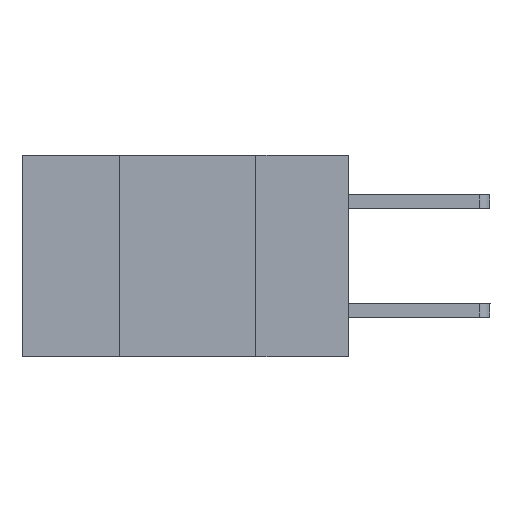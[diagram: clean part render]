
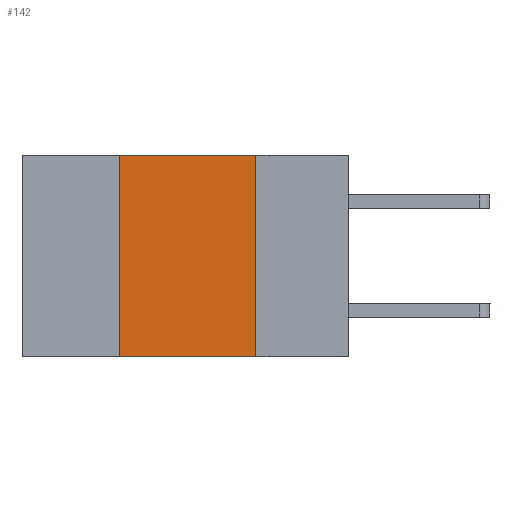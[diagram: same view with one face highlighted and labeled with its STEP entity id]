
A CAD part, left-side view. The second image highlights one B-rep face of the part: STEP entity #142.
In plain terms, the highlighted planar face has unit normal (-1, 0, 0).
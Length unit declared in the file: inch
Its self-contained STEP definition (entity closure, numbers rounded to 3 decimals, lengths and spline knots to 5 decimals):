
#65 = EDGE_CURVE ( 'NONE', #6121, #2360, #4379, .T. ) ;
#142 = ADVANCED_FACE ( 'NONE', ( #5683 ), #5788, .F. ) ;
#207 = LINE ( 'NONE', #7475, #9619 ) ;
#373 = EDGE_CURVE ( 'NONE', #6121, #1591, #207, .T. ) ;
#1591 = VERTEX_POINT ( 'NONE', #2227 ) ;
#1872 = CARTESIAN_POINT ( 'NONE',  ( 0., 0.17, -0.37 ) ) ;
#1943 = VECTOR ( 'NONE', #3594, 39.37008 ) ;
#2227 = CARTESIAN_POINT ( 'NONE',  ( 0., 0.42, 0. ) ) ;
#2360 = VERTEX_POINT ( 'NONE', #1872 ) ;
#2389 = VECTOR ( 'NONE', #4995, 39.37008 ) ;
#3249 = ORIENTED_EDGE ( 'NONE', *, *, #4396, .F. ) ;
#3594 = DIRECTION ( 'NONE',  ( 0., -1., 0. ) ) ;
#3815 = CARTESIAN_POINT ( 'NONE',  ( 0., 0.6, 0. ) ) ;
#3959 = CARTESIAN_POINT ( 'NONE',  ( 0., 0.17, -0.37 ) ) ;
#4371 = VECTOR ( 'NONE', #8391, 39.37008 ) ;
#4379 = LINE ( 'NONE', #9118, #2389 ) ;
#4396 = EDGE_CURVE ( 'NONE', #1591, #7978, #6060, .T. ) ;
#4505 = CARTESIAN_POINT ( 'NONE',  ( 0., 0.17, 0. ) ) ;
#4606 = DIRECTION ( 'NONE',  ( 0., 0., -1. ) ) ;
#4995 = DIRECTION ( 'NONE',  ( 0., -1., 0. ) ) ;
#5183 = DIRECTION ( 'NONE',  ( 0., 0., 1. ) ) ;
#5683 = FACE_OUTER_BOUND ( 'NONE', #9053, .T. ) ;
#5733 = AXIS2_PLACEMENT_3D ( 'NONE', #8387, #8668, #4606 ) ;
#5788 = PLANE ( 'NONE',  #5733 ) ;
#6060 = LINE ( 'NONE', #3815, #1943 ) ;
#6067 = ORIENTED_EDGE ( 'NONE', *, *, #65, .T. ) ;
#6121 = VERTEX_POINT ( 'NONE', #9562 ) ;
#6353 = EDGE_CURVE ( 'NONE', #7978, #2360, #8073, .T. ) ;
#6524 = ORIENTED_EDGE ( 'NONE', *, *, #6353, .F. ) ;
#6535 = ORIENTED_EDGE ( 'NONE', *, *, #373, .F. ) ;
#7475 = CARTESIAN_POINT ( 'NONE',  ( 0., 0.42, -0.37 ) ) ;
#7978 = VERTEX_POINT ( 'NONE', #4505 ) ;
#8073 = LINE ( 'NONE', #3959, #4371 ) ;
#8387 = CARTESIAN_POINT ( 'NONE',  ( 0., 0.6, 0. ) ) ;
#8391 = DIRECTION ( 'NONE',  ( 0., 0., -1. ) ) ;
#8668 = DIRECTION ( 'NONE',  ( 1., 0., 0. ) ) ;
#9053 = EDGE_LOOP ( 'NONE', ( #6524, #3249, #6535, #6067 ) ) ;
#9118 = CARTESIAN_POINT ( 'NONE',  ( 0., 0.6, -0.37 ) ) ;
#9562 = CARTESIAN_POINT ( 'NONE',  ( 0., 0.42, -0.37 ) ) ;
#9619 = VECTOR ( 'NONE', #5183, 39.37008 ) ;
